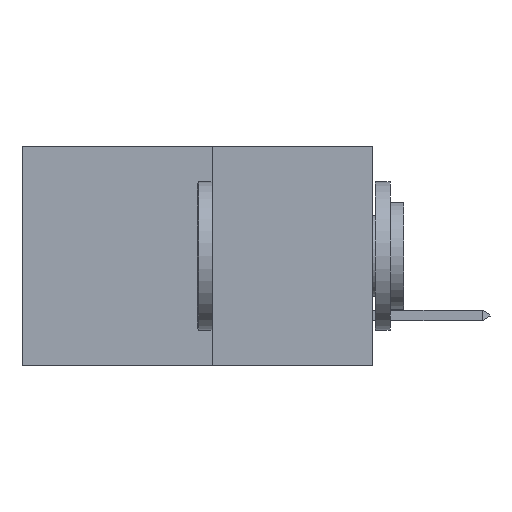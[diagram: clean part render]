
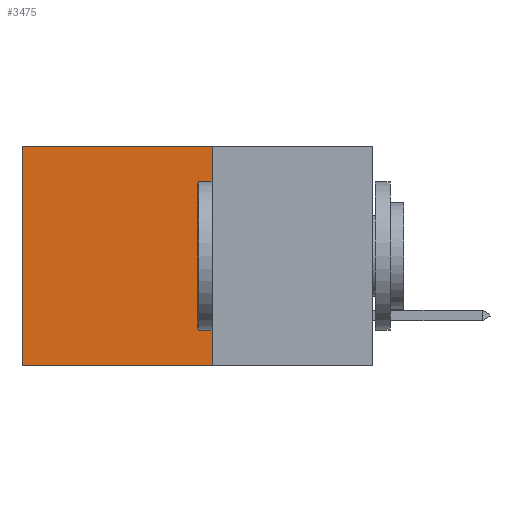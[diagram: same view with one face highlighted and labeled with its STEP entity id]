
A CAD part, left-side view. The second image highlights one B-rep face of the part: STEP entity #3475.
In plain terms, the highlighted planar face has unit normal (-1, 0, 0).
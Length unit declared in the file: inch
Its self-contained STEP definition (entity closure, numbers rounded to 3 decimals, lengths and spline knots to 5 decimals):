
#55 = DIRECTION ( 'NONE',  ( 0., 1., 0. ) ) ;
#472 = VERTEX_POINT ( 'NONE', #11586 ) ;
#563 = CARTESIAN_POINT ( 'NONE',  ( 0.277, 0.27, 0. ) ) ;
#905 = CARTESIAN_POINT ( 'NONE',  ( 0.277, 0.27, -0.37 ) ) ;
#1062 = VECTOR ( 'NONE', #14266, 39.37008 ) ;
#1754 = EDGE_CURVE ( 'NONE', #15922, #472, #4347, .T. ) ;
#3475 = ADVANCED_FACE ( 'NONE', ( #11378 ), #13382, .F. ) ;
#4271 = LINE ( 'NONE', #13153, #7945 ) ;
#4347 = LINE ( 'NONE', #563, #10083 ) ;
#4756 = LINE ( 'NONE', #8537, #7618 ) ;
#5401 = ORIENTED_EDGE ( 'NONE', *, *, #13942, .T. ) ;
#5852 = DIRECTION ( 'NONE',  ( 0., 0., -1. ) ) ;
#6963 = CARTESIAN_POINT ( 'NONE',  ( 0.277, 0.27, -0.37 ) ) ;
#7618 = VECTOR ( 'NONE', #15684, 39.37008 ) ;
#7945 = VECTOR ( 'NONE', #5852, 39.37008 ) ;
#8537 = CARTESIAN_POINT ( 'NONE',  ( 0.277, 0.27, -0.37 ) ) ;
#8797 = VERTEX_POINT ( 'NONE', #905 ) ;
#8813 = CARTESIAN_POINT ( 'NONE',  ( 0.277, 0.59, -0.37 ) ) ;
#8946 = VERTEX_POINT ( 'NONE', #8813 ) ;
#9307 = ORIENTED_EDGE ( 'NONE', *, *, #13917, .F. ) ;
#10083 = VECTOR ( 'NONE', #55, 39.37008 ) ;
#10827 = ORIENTED_EDGE ( 'NONE', *, *, #11561, .F. ) ;
#11136 = LINE ( 'NONE', #6963, #1062 ) ;
#11378 = FACE_OUTER_BOUND ( 'NONE', #13851, .T. ) ;
#11561 = EDGE_CURVE ( 'NONE', #15922, #8797, #4756, .T. ) ;
#11586 = CARTESIAN_POINT ( 'NONE',  ( 0.277, 0.59, 0. ) ) ;
#11867 = AXIS2_PLACEMENT_3D ( 'NONE', #13478, #13034, #12816 ) ;
#12212 = CARTESIAN_POINT ( 'NONE',  ( 0.277, 0.27, 0. ) ) ;
#12816 = DIRECTION ( 'NONE',  ( 0., 0., -1. ) ) ;
#12868 = ORIENTED_EDGE ( 'NONE', *, *, #1754, .T. ) ;
#13034 = DIRECTION ( 'NONE',  ( 1., 0., 0. ) ) ;
#13153 = CARTESIAN_POINT ( 'NONE',  ( 0.277, 0.59, -0.37 ) ) ;
#13382 = PLANE ( 'NONE',  #11867 ) ;
#13478 = CARTESIAN_POINT ( 'NONE',  ( 0.277, 0.27, -0.37 ) ) ;
#13851 = EDGE_LOOP ( 'NONE', ( #5401, #9307, #10827, #12868 ) ) ;
#13917 = EDGE_CURVE ( 'NONE', #8797, #8946, #11136, .T. ) ;
#13942 = EDGE_CURVE ( 'NONE', #472, #8946, #4271, .T. ) ;
#14266 = DIRECTION ( 'NONE',  ( 0., 1., 0. ) ) ;
#15684 = DIRECTION ( 'NONE',  ( 0., 0., -1. ) ) ;
#15922 = VERTEX_POINT ( 'NONE', #12212 ) ;
